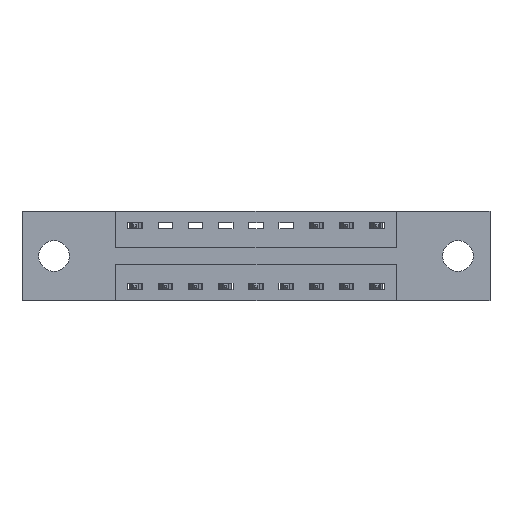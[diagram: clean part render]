
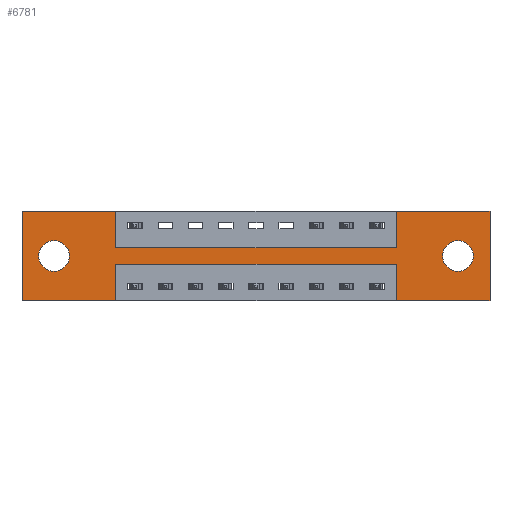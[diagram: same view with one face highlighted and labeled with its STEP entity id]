
A CAD part, front view. The second image highlights one B-rep face of the part: STEP entity #6781.
In plain terms, the highlighted planar face has unit normal (0, -1, 0).
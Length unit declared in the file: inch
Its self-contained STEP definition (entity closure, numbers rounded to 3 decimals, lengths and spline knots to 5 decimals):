
#12 = DIRECTION ( 'NONE',  ( 0., 0., 1. ) ) ;
#412 = EDGE_CURVE ( 'NONE', #3709, #6776, #6383, .T. ) ;
#573 = CARTESIAN_POINT ( 'NONE',  ( 0.3875, 0., -0.37 ) ) ;
#601 = CARTESIAN_POINT ( 'NONE',  ( 0., 0., 0. ) ) ;
#683 = EDGE_CURVE ( 'NONE', #9221, #6206, #1749, .T. ) ;
#712 = CARTESIAN_POINT ( 'NONE',  ( 0.1325, 0., -0.185 ) ) ;
#747 = EDGE_CURVE ( 'NONE', #6206, #9221, #2931, .T. ) ;
#1060 = VERTEX_POINT ( 'NONE', #7743 ) ;
#1078 = VERTEX_POINT ( 'NONE', #1173 ) ;
#1085 = EDGE_LOOP ( 'NONE', ( #5101, #1227 ) ) ;
#1148 = CARTESIAN_POINT ( 'NONE',  ( 0.3875, 0., -0.37 ) ) ;
#1168 = VECTOR ( 'NONE', #9470, 39.37008 ) ;
#1173 = CARTESIAN_POINT ( 'NONE',  ( 1.5475, 0., -0.37 ) ) ;
#1206 = DIRECTION ( 'NONE',  ( 0., 1., 0. ) ) ;
#1213 = VECTOR ( 'NONE', #12, 39.37008 ) ;
#1227 = ORIENTED_EDGE ( 'NONE', *, *, #10091, .T. ) ;
#1273 = CARTESIAN_POINT ( 'NONE',  ( 0.1325, 0., -0.185 ) ) ;
#1288 = VECTOR ( 'NONE', #1900, 39.37008 ) ;
#1323 = CARTESIAN_POINT ( 'NONE',  ( 1.5475, 0., -0.15 ) ) ;
#1352 = EDGE_CURVE ( 'NONE', #6476, #5522, #9811, .T. ) ;
#1360 = DIRECTION ( 'NONE',  ( 0., -1., 0. ) ) ;
#1437 = AXIS2_PLACEMENT_3D ( 'NONE', #1273, #4288, #5204 ) ;
#1492 = CARTESIAN_POINT ( 'NONE',  ( 0.1325, 0., -0.121 ) ) ;
#1749 = CIRCLE ( 'NONE', #1437, 0.064 ) ;
#1892 = VECTOR ( 'NONE', #3390, 39.37008 ) ;
#1900 = DIRECTION ( 'NONE',  ( 0., 0., -1. ) ) ;
#1920 = LINE ( 'NONE', #6432, #7936 ) ;
#2142 = CIRCLE ( 'NONE', #7742, 0.064 ) ;
#2209 = VERTEX_POINT ( 'NONE', #5353 ) ;
#2346 = EDGE_LOOP ( 'NONE', ( #6574, #5399 ) ) ;
#2391 = LINE ( 'NONE', #9448, #3518 ) ;
#2510 = EDGE_CURVE ( 'NONE', #5522, #2855, #4623, .T. ) ;
#2530 = ORIENTED_EDGE ( 'NONE', *, *, #5717, .F. ) ;
#2642 = CARTESIAN_POINT ( 'NONE',  ( 0.3875, 0., -0.22 ) ) ;
#2798 = DIRECTION ( 'NONE',  ( -1., 0., 0. ) ) ;
#2855 = VERTEX_POINT ( 'NONE', #6916 ) ;
#2877 = CARTESIAN_POINT ( 'NONE',  ( 0.3875, 0., -0.22 ) ) ;
#2893 = AXIS2_PLACEMENT_3D ( 'NONE', #6061, #1206, #6845 ) ;
#2931 = CIRCLE ( 'NONE', #3116, 0.064 ) ;
#2979 = EDGE_CURVE ( 'NONE', #6776, #8316, #7723, .T. ) ;
#3100 = ORIENTED_EDGE ( 'NONE', *, *, #6183, .F. ) ;
#3116 = AXIS2_PLACEMENT_3D ( 'NONE', #712, #9677, #8729 ) ;
#3332 = CARTESIAN_POINT ( 'NONE',  ( 0.3875, 0., 0. ) ) ;
#3390 = DIRECTION ( 'NONE',  ( 1., 0., 0. ) ) ;
#3503 = ORIENTED_EDGE ( 'NONE', *, *, #4337, .F. ) ;
#3504 = LINE ( 'NONE', #601, #7187 ) ;
#3518 = VECTOR ( 'NONE', #10177, 39.37008 ) ;
#3639 = VERTEX_POINT ( 'NONE', #10005 ) ;
#3647 = DIRECTION ( 'NONE',  ( -1., 0., 0. ) ) ;
#3709 = VERTEX_POINT ( 'NONE', #8585 ) ;
#3878 = DIRECTION ( 'NONE',  ( 0., 1., 0. ) ) ;
#3890 = VECTOR ( 'NONE', #3647, 39.37008 ) ;
#3918 = CARTESIAN_POINT ( 'NONE',  ( 1.5475, 0., 0. ) ) ;
#4038 = DIRECTION ( 'NONE',  ( 0., 0., 1. ) ) ;
#4096 = VERTEX_POINT ( 'NONE', #8400 ) ;
#4288 = DIRECTION ( 'NONE',  ( 0., 1., 0. ) ) ;
#4337 = EDGE_CURVE ( 'NONE', #2209, #1060, #9651, .T. ) ;
#4396 = VERTEX_POINT ( 'NONE', #5733 ) ;
#4500 = CARTESIAN_POINT ( 'NONE',  ( 1.5475, 0., -0.22 ) ) ;
#4623 = LINE ( 'NONE', #4913, #9904 ) ;
#4679 = EDGE_CURVE ( 'NONE', #4396, #3639, #8593, .T. ) ;
#4686 = VERTEX_POINT ( 'NONE', #4500 ) ;
#4863 = ORIENTED_EDGE ( 'NONE', *, *, #9818, .F. ) ;
#4886 = CARTESIAN_POINT ( 'NONE',  ( 1.935, 0., 0. ) ) ;
#4913 = CARTESIAN_POINT ( 'NONE',  ( 0., 0., -0.37 ) ) ;
#4972 = CARTESIAN_POINT ( 'NONE',  ( 0., 0., 0. ) ) ;
#5006 = EDGE_LOOP ( 'NONE', ( #8214, #5491, #8183, #4863, #3503, #2530, #5570, #7007, #8324, #3100, #7092, #5007 ) ) ;
#5007 = ORIENTED_EDGE ( 'NONE', *, *, #2510, .F. ) ;
#5101 = ORIENTED_EDGE ( 'NONE', *, *, #4679, .T. ) ;
#5204 = DIRECTION ( 'NONE',  ( 0., 0., 1. ) ) ;
#5242 = AXIS2_PLACEMENT_3D ( 'NONE', #5416, #1360, #6987 ) ;
#5353 = CARTESIAN_POINT ( 'NONE',  ( 1.935, 0., 0. ) ) ;
#5399 = ORIENTED_EDGE ( 'NONE', *, *, #683, .T. ) ;
#5416 = CARTESIAN_POINT ( 'NONE',  ( 0., 0., -0.37 ) ) ;
#5418 = VECTOR ( 'NONE', #9392, 39.37008 ) ;
#5491 = ORIENTED_EDGE ( 'NONE', *, *, #9877, .F. ) ;
#5514 = VERTEX_POINT ( 'NONE', #6248 ) ;
#5522 = VERTEX_POINT ( 'NONE', #573 ) ;
#5570 = ORIENTED_EDGE ( 'NONE', *, *, #2979, .F. ) ;
#5696 = DIRECTION ( 'NONE',  ( -1., 0., 0. ) ) ;
#5700 = VECTOR ( 'NONE', #9982, 39.37008 ) ;
#5717 = EDGE_CURVE ( 'NONE', #8316, #2209, #2391, .T. ) ;
#5733 = CARTESIAN_POINT ( 'NONE',  ( 1.8025, 0., -0.121 ) ) ;
#6061 = CARTESIAN_POINT ( 'NONE',  ( 1.8025, 0., -0.185 ) ) ;
#6114 = FACE_BOUND ( 'NONE', #1085, .T. ) ;
#6183 = EDGE_CURVE ( 'NONE', #5514, #4096, #3504, .T. ) ;
#6191 = PLANE ( 'NONE',  #5242 ) ;
#6206 = VERTEX_POINT ( 'NONE', #1492 ) ;
#6248 = CARTESIAN_POINT ( 'NONE',  ( 0., 0., 0. ) ) ;
#6383 = LINE ( 'NONE', #7326, #1892 ) ;
#6394 = EDGE_CURVE ( 'NONE', #4096, #3709, #9494, .T. ) ;
#6432 = CARTESIAN_POINT ( 'NONE',  ( 1.5475, 0., -0.37 ) ) ;
#6476 = VERTEX_POINT ( 'NONE', #2642 ) ;
#6574 = ORIENTED_EDGE ( 'NONE', *, *, #747, .T. ) ;
#6776 = VERTEX_POINT ( 'NONE', #1323 ) ;
#6781 = ADVANCED_FACE ( 'NONE', ( #6114, #7653, #9617 ), #6191, .T. ) ;
#6845 = DIRECTION ( 'NONE',  ( 0., 0., -1. ) ) ;
#6916 = CARTESIAN_POINT ( 'NONE',  ( 0., 0., -0.37 ) ) ;
#6987 = DIRECTION ( 'NONE',  ( 0., 0., -1. ) ) ;
#7007 = ORIENTED_EDGE ( 'NONE', *, *, #412, .F. ) ;
#7092 = ORIENTED_EDGE ( 'NONE', *, *, #9082, .F. ) ;
#7187 = VECTOR ( 'NONE', #7797, 39.37008 ) ;
#7207 = LINE ( 'NONE', #7476, #8695 ) ;
#7326 = CARTESIAN_POINT ( 'NONE',  ( 0.3875, 0., -0.15 ) ) ;
#7476 = CARTESIAN_POINT ( 'NONE',  ( 0., 0., -0.37 ) ) ;
#7653 = FACE_BOUND ( 'NONE', #2346, .T. ) ;
#7723 = LINE ( 'NONE', #8507, #5700 ) ;
#7742 = AXIS2_PLACEMENT_3D ( 'NONE', #8492, #3878, #9238 ) ;
#7743 = CARTESIAN_POINT ( 'NONE',  ( 1.935, 0., -0.37 ) ) ;
#7797 = DIRECTION ( 'NONE',  ( 1., 0., 0. ) ) ;
#7936 = VECTOR ( 'NONE', #4038, 39.37008 ) ;
#8167 = CARTESIAN_POINT ( 'NONE',  ( 0.1325, 0., -0.249 ) ) ;
#8183 = ORIENTED_EDGE ( 'NONE', *, *, #8407, .F. ) ;
#8214 = ORIENTED_EDGE ( 'NONE', *, *, #1352, .F. ) ;
#8316 = VERTEX_POINT ( 'NONE', #3918 ) ;
#8324 = ORIENTED_EDGE ( 'NONE', *, *, #6394, .F. ) ;
#8400 = CARTESIAN_POINT ( 'NONE',  ( 0.3875, 0., 0. ) ) ;
#8407 = EDGE_CURVE ( 'NONE', #1078, #4686, #1920, .T. ) ;
#8492 = CARTESIAN_POINT ( 'NONE',  ( 1.8025, 0., -0.185 ) ) ;
#8507 = CARTESIAN_POINT ( 'NONE',  ( 1.5475, 0., 0. ) ) ;
#8585 = CARTESIAN_POINT ( 'NONE',  ( 0.3875, 0., -0.15 ) ) ;
#8593 = CIRCLE ( 'NONE', #2893, 0.064 ) ;
#8695 = VECTOR ( 'NONE', #2798, 39.37008 ) ;
#8729 = DIRECTION ( 'NONE',  ( 0., 0., 1. ) ) ;
#9082 = EDGE_CURVE ( 'NONE', #2855, #5514, #9534, .T. ) ;
#9221 = VERTEX_POINT ( 'NONE', #8167 ) ;
#9238 = DIRECTION ( 'NONE',  ( 0., 0., -1. ) ) ;
#9392 = DIRECTION ( 'NONE',  ( 0., 0., -1. ) ) ;
#9448 = CARTESIAN_POINT ( 'NONE',  ( 0., 0., 0. ) ) ;
#9470 = DIRECTION ( 'NONE',  ( 0., 0., -1. ) ) ;
#9494 = LINE ( 'NONE', #3332, #1168 ) ;
#9534 = LINE ( 'NONE', #4972, #1213 ) ;
#9617 = FACE_OUTER_BOUND ( 'NONE', #5006, .T. ) ;
#9651 = LINE ( 'NONE', #4886, #5418 ) ;
#9677 = DIRECTION ( 'NONE',  ( 0., 1., 0. ) ) ;
#9811 = LINE ( 'NONE', #1148, #1288 ) ;
#9818 = EDGE_CURVE ( 'NONE', #1060, #1078, #7207, .T. ) ;
#9877 = EDGE_CURVE ( 'NONE', #4686, #6476, #9964, .T. ) ;
#9904 = VECTOR ( 'NONE', #5696, 39.37008 ) ;
#9964 = LINE ( 'NONE', #2877, #3890 ) ;
#9982 = DIRECTION ( 'NONE',  ( 0., 0., 1. ) ) ;
#10005 = CARTESIAN_POINT ( 'NONE',  ( 1.8025, 0., -0.249 ) ) ;
#10091 = EDGE_CURVE ( 'NONE', #3639, #4396, #2142, .T. ) ;
#10177 = DIRECTION ( 'NONE',  ( 1., 0., 0. ) ) ;
